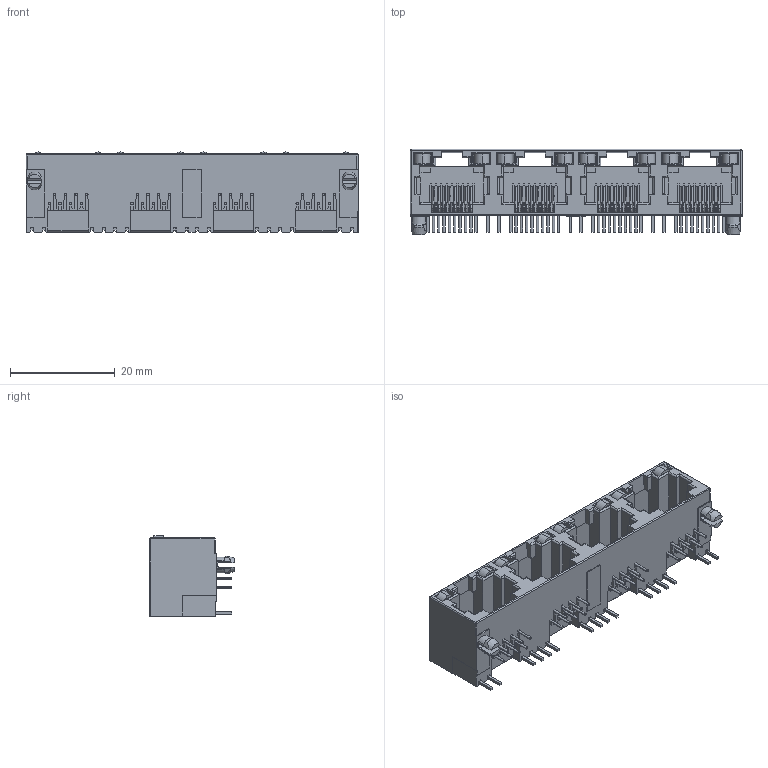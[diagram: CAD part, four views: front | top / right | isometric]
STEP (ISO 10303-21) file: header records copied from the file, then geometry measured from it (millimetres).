
FILE_DESCRIPTION (( 'STEP AP203' ), '1' );
FILE_NAME ('J67048822P11011.STEP', '2020-03-20T12:10:38', ( '' ), ( '' ), 'SwSTEP 2.0', 'SolidWorks 2016', '' );
FILE_SCHEMA (( 'CONFIG_CONTROL_DESIGN' ));
Length unit declared in the file: millimetre
Products named in the file (5): 67 Contacts; 67 LED RH_1-Yellow; 67 LED LH_1-Yellow; J67048822P11011; 67 Insulator
Assembly tree (13 placements, depth 2):
  J67048822P11011
    67 Insulator
    67 Contacts  x4
    67 LED LH_1-Yellow  x4
    67 LED RH_1-Yellow  x4
Bounding box: 63.3 x 16.25 x 15.28 mm (x, y, z)
Volume: 5159.3 mm3; surface area: 11572.8 mm2
Topology: 41 solids, 41 shells, 2465 faces, 6544 edges, 4096 vertices
Faces by surface type: plane 1781, cylinder 476, bspline 200, cone 8
Entity records: 62393 total; most frequent: CARTESIAN_POINT 12221, ORIENTED_EDGE 10780, DIRECTION 9576, EDGE_CURVE 5390, VECTOR 4682, LINE 4682, VERTEX_POINT 3364, AXIS2_PLACEMENT_3D 2447
